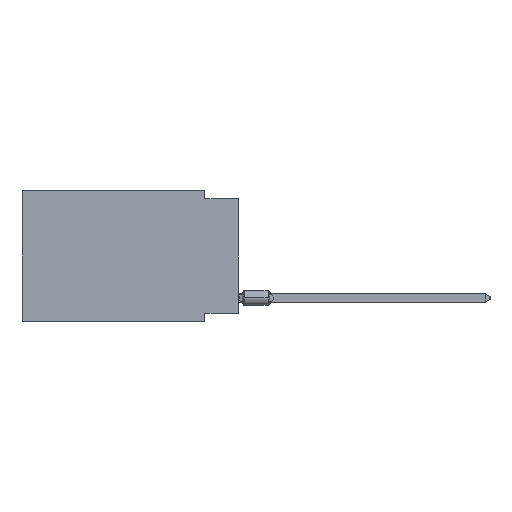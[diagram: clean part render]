
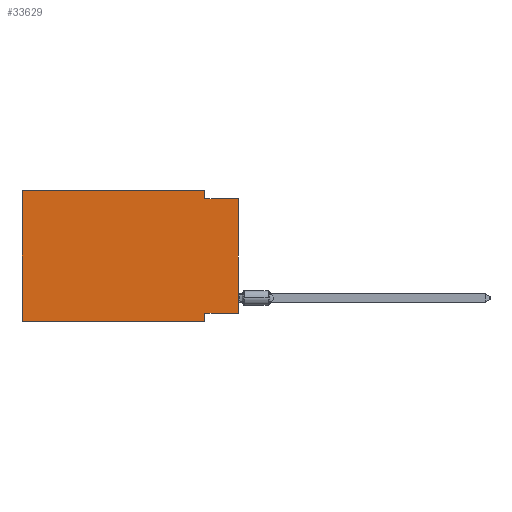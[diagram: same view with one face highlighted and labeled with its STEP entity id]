
A CAD part, left-side view. The second image highlights one B-rep face of the part: STEP entity #33629.
In plain terms, the highlighted planar face has unit normal (-1, 0, 0).
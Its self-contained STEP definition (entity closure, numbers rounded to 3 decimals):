
#3949 = ORIENTED_EDGE ( 'NONE', *, *, #52049, .F. ) ;
#4031 = ORIENTED_EDGE ( 'NONE', *, *, #33630, .F. ) ;
#4071 = VECTOR ( 'NONE', #31074, 1000. ) ;
#4641 = VERTEX_POINT ( 'NONE', #11205 ) ;
#5204 = LINE ( 'NONE', #28547, #36699 ) ;
#6246 = LINE ( 'NONE', #38819, #51246 ) ;
#8167 = EDGE_CURVE ( 'NONE', #25149, #31374, #30301, .T. ) ;
#8431 = CARTESIAN_POINT ( 'NONE',  ( 0., 16.383, 0. ) ) ;
#8597 = AXIS2_PLACEMENT_3D ( 'NONE', #8431, #22569, #49110 ) ;
#8675 = VECTOR ( 'NONE', #37288, 1000. ) ;
#9328 = VECTOR ( 'NONE', #18965, 1000. ) ;
#11178 = DIRECTION ( 'NONE',  ( 0., 0., 1. ) ) ;
#11205 = CARTESIAN_POINT ( 'NONE',  ( 0., 2.54, -9.906 ) ) ;
#11388 = ORIENTED_EDGE ( 'NONE', *, *, #23980, .T. ) ;
#11492 = EDGE_CURVE ( 'NONE', #31374, #4641, #6246, .T. ) ;
#12138 = VERTEX_POINT ( 'NONE', #60000 ) ;
#13336 = CARTESIAN_POINT ( 'NONE',  ( 0., 2.54, 0. ) ) ;
#14570 = CARTESIAN_POINT ( 'NONE',  ( 0., 0., -9.271 ) ) ;
#15474 = DIRECTION ( 'NONE',  ( 0., 0., -1. ) ) ;
#15762 = LINE ( 'NONE', #34494, #4071 ) ;
#16008 = EDGE_LOOP ( 'NONE', ( #11388, #39309, #3949, #33461, #4031, #18397, #37969, #32530 ) ) ;
#17643 = VECTOR ( 'NONE', #11178, 1000. ) ;
#18397 = ORIENTED_EDGE ( 'NONE', *, *, #57393, .T. ) ;
#18548 = LINE ( 'NONE', #46502, #8675 ) ;
#18965 = DIRECTION ( 'NONE',  ( 0., -1., 0. ) ) ;
#22569 = DIRECTION ( 'NONE',  ( 1., 0., 0. ) ) ;
#22679 = CARTESIAN_POINT ( 'NONE',  ( 0., 2.54, -9.271 ) ) ;
#23980 = EDGE_CURVE ( 'NONE', #25149, #12138, #44025, .T. ) ;
#25137 = FACE_OUTER_BOUND ( 'NONE', #16008, .T. ) ;
#25149 = VERTEX_POINT ( 'NONE', #14570 ) ;
#26588 = VERTEX_POINT ( 'NONE', #27947 ) ;
#27947 = CARTESIAN_POINT ( 'NONE',  ( 0., 16.383, 0. ) ) ;
#28547 = CARTESIAN_POINT ( 'NONE',  ( 0., 0., -0.635 ) ) ;
#29325 = EDGE_CURVE ( 'NONE', #43121, #12138, #5204, .T. ) ;
#30301 = LINE ( 'NONE', #53045, #48258 ) ;
#30760 = CARTESIAN_POINT ( 'NONE',  ( 0., 2.54, -0.635 ) ) ;
#31074 = DIRECTION ( 'NONE',  ( 0., -1., 0. ) ) ;
#31374 = VERTEX_POINT ( 'NONE', #22679 ) ;
#31786 = DIRECTION ( 'NONE',  ( 0., 0., 1. ) ) ;
#32530 = ORIENTED_EDGE ( 'NONE', *, *, #8167, .F. ) ;
#33307 = VERTEX_POINT ( 'NONE', #35345 ) ;
#33461 = ORIENTED_EDGE ( 'NONE', *, *, #40672, .F. ) ;
#33629 = ADVANCED_FACE ( 'NONE', ( #25137 ), #39289, .F. ) ;
#33630 = EDGE_CURVE ( 'NONE', #33307, #26588, #50516, .T. ) ;
#34494 = CARTESIAN_POINT ( 'NONE',  ( 0., 16.383, -9.906 ) ) ;
#35345 = CARTESIAN_POINT ( 'NONE',  ( 0., 16.383, -9.906 ) ) ;
#35721 = CARTESIAN_POINT ( 'NONE',  ( 0., 0., 0. ) ) ;
#36699 = VECTOR ( 'NONE', #41778, 1000. ) ;
#37288 = DIRECTION ( 'NONE',  ( 0., 0., -1. ) ) ;
#37969 = ORIENTED_EDGE ( 'NONE', *, *, #11492, .F. ) ;
#38819 = CARTESIAN_POINT ( 'NONE',  ( 0., 2.54, -9.906 ) ) ;
#38920 = DIRECTION ( 'NONE',  ( 0., 1., 0. ) ) ;
#39289 = PLANE ( 'NONE',  #8597 ) ;
#39309 = ORIENTED_EDGE ( 'NONE', *, *, #29325, .F. ) ;
#39582 = CARTESIAN_POINT ( 'NONE',  ( 0., 16.383, 0. ) ) ;
#40672 = EDGE_CURVE ( 'NONE', #26588, #60022, #56107, .T. ) ;
#41778 = DIRECTION ( 'NONE',  ( 0., -1., 0. ) ) ;
#42962 = VECTOR ( 'NONE', #31786, 1000. ) ;
#43121 = VERTEX_POINT ( 'NONE', #30760 ) ;
#44025 = LINE ( 'NONE', #35721, #17643 ) ;
#46502 = CARTESIAN_POINT ( 'NONE',  ( 0., 2.54, 0. ) ) ;
#48258 = VECTOR ( 'NONE', #38920, 1000. ) ;
#49110 = DIRECTION ( 'NONE',  ( 0., 0., -1. ) ) ;
#50516 = LINE ( 'NONE', #39582, #42962 ) ;
#51246 = VECTOR ( 'NONE', #15474, 1000. ) ;
#52049 = EDGE_CURVE ( 'NONE', #60022, #43121, #18548, .T. ) ;
#53045 = CARTESIAN_POINT ( 'NONE',  ( 0., 0., -9.271 ) ) ;
#56107 = LINE ( 'NONE', #60713, #9328 ) ;
#57393 = EDGE_CURVE ( 'NONE', #33307, #4641, #15762, .T. ) ;
#60000 = CARTESIAN_POINT ( 'NONE',  ( 0., 0., -0.635 ) ) ;
#60022 = VERTEX_POINT ( 'NONE', #13336 ) ;
#60713 = CARTESIAN_POINT ( 'NONE',  ( 0., 16.383, 0. ) ) ;
